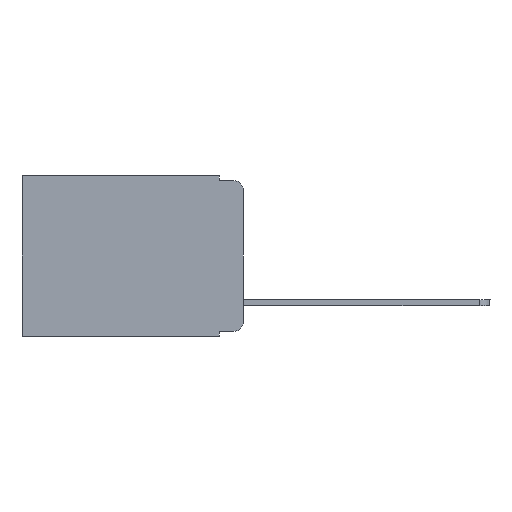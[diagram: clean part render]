
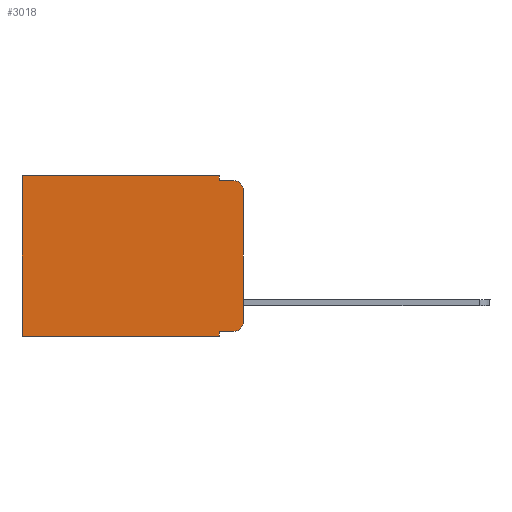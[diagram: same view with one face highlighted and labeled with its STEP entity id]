
A CAD part, left-side view. The second image highlights one B-rep face of the part: STEP entity #3018.
In plain terms, the highlighted planar face has unit normal (-1, 0, 0).
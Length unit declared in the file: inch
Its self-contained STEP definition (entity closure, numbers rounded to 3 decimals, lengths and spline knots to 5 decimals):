
#6 = VECTOR ( 'NONE', #15309, 39.37008 ) ;
#309 = DIRECTION ( 'NONE',  ( -1., 0., 0. ) ) ;
#438 = AXIS2_PLACEMENT_3D ( 'NONE', #11844, #12064, #7260 ) ;
#826 = EDGE_CURVE ( 'NONE', #5206, #6235, #15306, .T. ) ;
#880 = ORIENTED_EDGE ( 'NONE', *, *, #5879, .F. ) ;
#1271 = LINE ( 'NONE', #1431, #15716 ) ;
#1400 = LINE ( 'NONE', #7284, #2914 ) ;
#1431 = CARTESIAN_POINT ( 'NONE',  ( 0.298, 0., 0. ) ) ;
#1581 = VECTOR ( 'NONE', #1624, 39.37008 ) ;
#1624 = DIRECTION ( 'NONE',  ( 0., 0., -1. ) ) ;
#1763 = LINE ( 'NONE', #5620, #2089 ) ;
#2089 = VECTOR ( 'NONE', #14215, 39.37008 ) ;
#2377 = ORIENTED_EDGE ( 'NONE', *, *, #14819, .T. ) ;
#2431 = LINE ( 'NONE', #12243, #9081 ) ;
#2550 = DIRECTION ( 'NONE',  ( 0., 0., -1. ) ) ;
#2821 = CARTESIAN_POINT ( 'NONE',  ( 0.298, 0.473, 0. ) ) ;
#2868 = CARTESIAN_POINT ( 'NONE',  ( 0.298, 0.051, -0.343 ) ) ;
#2914 = VECTOR ( 'NONE', #12168, 39.37008 ) ;
#2956 = VERTEX_POINT ( 'NONE', #10683 ) ;
#3018 = ADVANCED_FACE ( 'NONE', ( #13151 ), #4634, .F. ) ;
#3310 = CARTESIAN_POINT ( 'NONE',  ( 0.298, 0.02, -0.333 ) ) ;
#3357 = VERTEX_POINT ( 'NONE', #3310 ) ;
#3448 = CARTESIAN_POINT ( 'NONE',  ( 0.298, 0.473, -0.343 ) ) ;
#3593 = EDGE_CURVE ( 'NONE', #6615, #12237, #1763, .T. ) ;
#3984 = ORIENTED_EDGE ( 'NONE', *, *, #10262, .T. ) ;
#4010 = ORIENTED_EDGE ( 'NONE', *, *, #10273, .F. ) ;
#4196 = EDGE_LOOP ( 'NONE', ( #9508, #9317, #880, #7877, #8347, #3984, #10114, #4010, #6993, #2377 ) ) ;
#4634 = PLANE ( 'NONE',  #11268 ) ;
#4773 = CARTESIAN_POINT ( 'NONE',  ( 0.298, 0.473, 0. ) ) ;
#5161 = EDGE_CURVE ( 'NONE', #7991, #5426, #1271, .T. ) ;
#5206 = VERTEX_POINT ( 'NONE', #10992 ) ;
#5320 = LINE ( 'NONE', #2821, #14140 ) ;
#5398 = CARTESIAN_POINT ( 'NONE',  ( 0.298, 0.051, -0.333 ) ) ;
#5426 = VERTEX_POINT ( 'NONE', #4773 ) ;
#5456 = AXIS2_PLACEMENT_3D ( 'NONE', #11300, #309, #2550 ) ;
#5506 = EDGE_CURVE ( 'NONE', #5731, #3357, #2431, .T. ) ;
#5620 = CARTESIAN_POINT ( 'NONE',  ( 0.298, 0., -0.343 ) ) ;
#5665 = CARTESIAN_POINT ( 'NONE',  ( 0.298, 0., 0. ) ) ;
#5731 = VERTEX_POINT ( 'NONE', #5398 ) ;
#5879 = EDGE_CURVE ( 'NONE', #2956, #6235, #6921, .T. ) ;
#6235 = VERTEX_POINT ( 'NONE', #7882 ) ;
#6308 = DIRECTION ( 'NONE',  ( 0., -1., 0. ) ) ;
#6610 = CARTESIAN_POINT ( 'NONE',  ( 0.298, 0.051, 0. ) ) ;
#6615 = VERTEX_POINT ( 'NONE', #2868 ) ;
#6759 = CIRCLE ( 'NONE', #5456, 0.02 ) ;
#6921 = LINE ( 'NONE', #9501, #14972 ) ;
#6993 = ORIENTED_EDGE ( 'NONE', *, *, #5506, .T. ) ;
#7145 = DIRECTION ( 'NONE',  ( 0., 0., -1. ) ) ;
#7260 = DIRECTION ( 'NONE',  ( 0., 0., -1. ) ) ;
#7284 = CARTESIAN_POINT ( 'NONE',  ( 0.298, 0.051, 0. ) ) ;
#7584 = VERTEX_POINT ( 'NONE', #8279 ) ;
#7877 = ORIENTED_EDGE ( 'NONE', *, *, #15724, .F. ) ;
#7882 = CARTESIAN_POINT ( 'NONE',  ( 0.298, 0.02, -0.01 ) ) ;
#7991 = VERTEX_POINT ( 'NONE', #14432 ) ;
#8279 = CARTESIAN_POINT ( 'NONE',  ( 0.298, 0., -0.313 ) ) ;
#8347 = ORIENTED_EDGE ( 'NONE', *, *, #5161, .T. ) ;
#9081 = VECTOR ( 'NONE', #6308, 39.37008 ) ;
#9317 = ORIENTED_EDGE ( 'NONE', *, *, #826, .T. ) ;
#9501 = CARTESIAN_POINT ( 'NONE',  ( 0.298, 0.051, -0.01 ) ) ;
#9508 = ORIENTED_EDGE ( 'NONE', *, *, #12483, .F. ) ;
#9544 = CARTESIAN_POINT ( 'NONE',  ( 0.298, 0., 0. ) ) ;
#9789 = DIRECTION ( 'NONE',  ( 0., 1., 0. ) ) ;
#10114 = ORIENTED_EDGE ( 'NONE', *, *, #3593, .F. ) ;
#10236 = LINE ( 'NONE', #6610, #1581 ) ;
#10262 = EDGE_CURVE ( 'NONE', #5426, #12237, #5320, .T. ) ;
#10273 = EDGE_CURVE ( 'NONE', #5731, #6615, #10236, .T. ) ;
#10683 = CARTESIAN_POINT ( 'NONE',  ( 0.298, 0.051, -0.01 ) ) ;
#10992 = CARTESIAN_POINT ( 'NONE',  ( 0.298, 0., -0.03 ) ) ;
#11268 = AXIS2_PLACEMENT_3D ( 'NONE', #9544, #13226, #7145 ) ;
#11300 = CARTESIAN_POINT ( 'NONE',  ( 0.298, 0.02, -0.313 ) ) ;
#11844 = CARTESIAN_POINT ( 'NONE',  ( 0.298, 0.02, -0.03 ) ) ;
#12064 = DIRECTION ( 'NONE',  ( -1., 0., 0. ) ) ;
#12168 = DIRECTION ( 'NONE',  ( 0., 0., -1. ) ) ;
#12237 = VERTEX_POINT ( 'NONE', #3448 ) ;
#12243 = CARTESIAN_POINT ( 'NONE',  ( 0.298, 0.051, -0.333 ) ) ;
#12483 = EDGE_CURVE ( 'NONE', #5206, #7584, #15379, .T. ) ;
#13151 = FACE_OUTER_BOUND ( 'NONE', #4196, .T. ) ;
#13226 = DIRECTION ( 'NONE',  ( 1., 0., 0. ) ) ;
#13751 = DIRECTION ( 'NONE',  ( 0., 0., -1. ) ) ;
#14140 = VECTOR ( 'NONE', #13751, 39.37008 ) ;
#14215 = DIRECTION ( 'NONE',  ( 0., 1., 0. ) ) ;
#14432 = CARTESIAN_POINT ( 'NONE',  ( 0.298, 0.051, 0. ) ) ;
#14819 = EDGE_CURVE ( 'NONE', #3357, #7584, #6759, .T. ) ;
#14972 = VECTOR ( 'NONE', #15750, 39.37008 ) ;
#15306 = CIRCLE ( 'NONE', #438, 0.02 ) ;
#15309 = DIRECTION ( 'NONE',  ( 0., 0., -1. ) ) ;
#15379 = LINE ( 'NONE', #5665, #6 ) ;
#15716 = VECTOR ( 'NONE', #9789, 39.37008 ) ;
#15724 = EDGE_CURVE ( 'NONE', #7991, #2956, #1400, .T. ) ;
#15750 = DIRECTION ( 'NONE',  ( 0., -1., 0. ) ) ;
